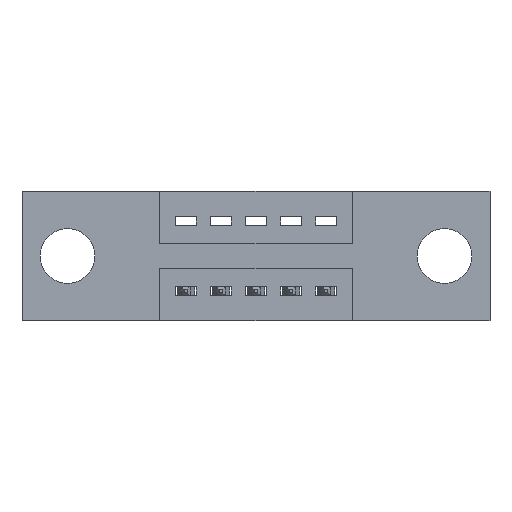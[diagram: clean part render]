
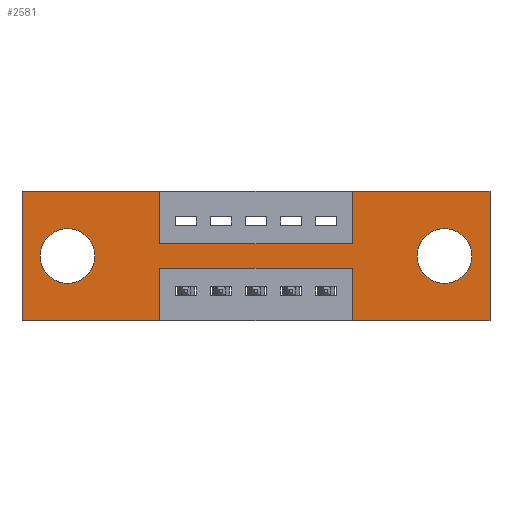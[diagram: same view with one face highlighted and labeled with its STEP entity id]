
A CAD part, front view. The second image highlights one B-rep face of the part: STEP entity #2581.
In plain terms, the highlighted planar face has unit normal (0, -1, 0).
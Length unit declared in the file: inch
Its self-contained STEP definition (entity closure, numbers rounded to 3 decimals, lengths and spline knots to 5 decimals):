
#15 = CARTESIAN_POINT ( 'NONE',  ( 0.13, 0., -0.263 ) ) ;
#109 = EDGE_CURVE ( 'NONE', #8626, #171, #8710, .T. ) ;
#113 = LINE ( 'NONE', #3577, #8083 ) ;
#143 = FACE_BOUND ( 'NONE', #386, .T. ) ;
#150 = ORIENTED_EDGE ( 'NONE', *, *, #3169, .F. ) ;
#171 = VERTEX_POINT ( 'NONE', #7213 ) ;
#253 = VERTEX_POINT ( 'NONE', #6100 ) ;
#336 = VERTEX_POINT ( 'NONE', #4728 ) ;
#356 = VERTEX_POINT ( 'NONE', #8043 ) ;
#372 = DIRECTION ( 'NONE',  ( 1., 0., 0. ) ) ;
#386 = EDGE_LOOP ( 'NONE', ( #6380, #6823 ) ) ;
#454 = VERTEX_POINT ( 'NONE', #6214 ) ;
#799 = VERTEX_POINT ( 'NONE', #6121 ) ;
#828 = LINE ( 'NONE', #1223, #1150 ) ;
#867 = ORIENTED_EDGE ( 'NONE', *, *, #2726, .F. ) ;
#883 = CARTESIAN_POINT ( 'NONE',  ( 0.9425, 0., 0. ) ) ;
#956 = DIRECTION ( 'NONE',  ( 0., 0., 1. ) ) ;
#1019 = DIRECTION ( 'NONE',  ( 0., 1., 0. ) ) ;
#1147 = CARTESIAN_POINT ( 'NONE',  ( 0.9425, 0., -0.37 ) ) ;
#1150 = VECTOR ( 'NONE', #3810, 39.37008 ) ;
#1153 = CARTESIAN_POINT ( 'NONE',  ( 0., 0., 0. ) ) ;
#1200 = AXIS2_PLACEMENT_3D ( 'NONE', #6505, #1019, #956 ) ;
#1213 = DIRECTION ( 'NONE',  ( -1., 0., 0. ) ) ;
#1223 = CARTESIAN_POINT ( 'NONE',  ( 0.3925, 0., -0.22 ) ) ;
#1631 = EDGE_CURVE ( 'NONE', #1821, #336, #8228, .T. ) ;
#1748 = CARTESIAN_POINT ( 'NONE',  ( 0., 0., 0. ) ) ;
#1821 = VERTEX_POINT ( 'NONE', #4134 ) ;
#1927 = CARTESIAN_POINT ( 'NONE',  ( 0.3925, 0., -0.22 ) ) ;
#2043 = CIRCLE ( 'NONE', #7856, 0.078 ) ;
#2061 = DIRECTION ( 'NONE',  ( 0., 0., -1. ) ) ;
#2185 = EDGE_LOOP ( 'NONE', ( #150, #3767, #7051, #867, #5070, #3225, #2313, #6167, #3788, #2284, #3753, #7090 ) ) ;
#2240 = DIRECTION ( 'NONE',  ( 0., 0., 1. ) ) ;
#2284 = ORIENTED_EDGE ( 'NONE', *, *, #5290, .F. ) ;
#2313 = ORIENTED_EDGE ( 'NONE', *, *, #2867, .F. ) ;
#2475 = VECTOR ( 'NONE', #4368, 39.37008 ) ;
#2581 = ADVANCED_FACE ( 'NONE', ( #143, #7480, #3750 ), #8185, .T. ) ;
#2722 = CARTESIAN_POINT ( 'NONE',  ( 0.3925, 0., -0.37 ) ) ;
#2726 = EDGE_CURVE ( 'NONE', #8223, #3061, #7687, .T. ) ;
#2732 = DIRECTION ( 'NONE',  ( 0., 1., 0. ) ) ;
#2829 = DIRECTION ( 'NONE',  ( 0., 0., -1. ) ) ;
#2867 = EDGE_CURVE ( 'NONE', #5758, #8626, #7140, .T. ) ;
#2986 = DIRECTION ( 'NONE',  ( 0., 0., -1. ) ) ;
#3061 = VERTEX_POINT ( 'NONE', #6664 ) ;
#3068 = LINE ( 'NONE', #3722, #8256 ) ;
#3169 = EDGE_CURVE ( 'NONE', #3504, #6821, #8399, .T. ) ;
#3225 = ORIENTED_EDGE ( 'NONE', *, *, #109, .F. ) ;
#3300 = LINE ( 'NONE', #6414, #7873 ) ;
#3504 = VERTEX_POINT ( 'NONE', #1927 ) ;
#3577 = CARTESIAN_POINT ( 'NONE',  ( 0.3925, 0., -0.15 ) ) ;
#3605 = LINE ( 'NONE', #5418, #8680 ) ;
#3722 = CARTESIAN_POINT ( 'NONE',  ( 0., 0., 0. ) ) ;
#3750 = FACE_OUTER_BOUND ( 'NONE', #2185, .T. ) ;
#3753 = ORIENTED_EDGE ( 'NONE', *, *, #7969, .F. ) ;
#3767 = ORIENTED_EDGE ( 'NONE', *, *, #8628, .F. ) ;
#3788 = ORIENTED_EDGE ( 'NONE', *, *, #4035, .F. ) ;
#3810 = DIRECTION ( 'NONE',  ( -1., 0., 0. ) ) ;
#3904 = CARTESIAN_POINT ( 'NONE',  ( 0.3925, 0., 0. ) ) ;
#3978 = VERTEX_POINT ( 'NONE', #5642 ) ;
#4035 = EDGE_CURVE ( 'NONE', #5348, #454, #3300, .T. ) ;
#4040 = EDGE_CURVE ( 'NONE', #454, #5758, #113, .T. ) ;
#4134 = CARTESIAN_POINT ( 'NONE',  ( 1.205, 0., -0.107 ) ) ;
#4186 = VECTOR ( 'NONE', #2240, 39.37008 ) ;
#4225 = AXIS2_PLACEMENT_3D ( 'NONE', #7318, #5202, #5286 ) ;
#4337 = LINE ( 'NONE', #1147, #8250 ) ;
#4368 = DIRECTION ( 'NONE',  ( 1., 0., 0. ) ) ;
#4728 = CARTESIAN_POINT ( 'NONE',  ( 1.205, 0., -0.263 ) ) ;
#4789 = EDGE_CURVE ( 'NONE', #6821, #3978, #7316, .T. ) ;
#4800 = EDGE_CURVE ( 'NONE', #171, #8223, #3605, .T. ) ;
#4844 = DIRECTION ( 'NONE',  ( 0., -1., 0. ) ) ;
#4941 = CARTESIAN_POINT ( 'NONE',  ( 0.13, 0., -0.185 ) ) ;
#5070 = ORIENTED_EDGE ( 'NONE', *, *, #4800, .F. ) ;
#5202 = DIRECTION ( 'NONE',  ( 0., 1., 0. ) ) ;
#5286 = DIRECTION ( 'NONE',  ( 0., 0., -1. ) ) ;
#5287 = CARTESIAN_POINT ( 'NONE',  ( 0., 0., -0.37 ) ) ;
#5290 = EDGE_CURVE ( 'NONE', #356, #5348, #6994, .T. ) ;
#5348 = VERTEX_POINT ( 'NONE', #3904 ) ;
#5418 = CARTESIAN_POINT ( 'NONE',  ( 1.335, 0., 0. ) ) ;
#5642 = CARTESIAN_POINT ( 'NONE',  ( 0., 0., -0.37 ) ) ;
#5758 = VERTEX_POINT ( 'NONE', #6337 ) ;
#5895 = VECTOR ( 'NONE', #1213, 39.37008 ) ;
#6072 = CIRCLE ( 'NONE', #1200, 0.078 ) ;
#6100 = CARTESIAN_POINT ( 'NONE',  ( 0.9425, 0., -0.22 ) ) ;
#6119 = CARTESIAN_POINT ( 'NONE',  ( 1.205, 0., -0.185 ) ) ;
#6121 = CARTESIAN_POINT ( 'NONE',  ( 0.13, 0., -0.107 ) ) ;
#6167 = ORIENTED_EDGE ( 'NONE', *, *, #4040, .F. ) ;
#6205 = VECTOR ( 'NONE', #2061, 39.37008 ) ;
#6214 = CARTESIAN_POINT ( 'NONE',  ( 0.3925, 0., -0.15 ) ) ;
#6236 = EDGE_LOOP ( 'NONE', ( #7913, #6737 ) ) ;
#6259 = AXIS2_PLACEMENT_3D ( 'NONE', #8208, #4844, #2829 ) ;
#6337 = CARTESIAN_POINT ( 'NONE',  ( 0.9425, 0., -0.15 ) ) ;
#6372 = DIRECTION ( 'NONE',  ( 0., 0., 1. ) ) ;
#6380 = ORIENTED_EDGE ( 'NONE', *, *, #1631, .T. ) ;
#6414 = CARTESIAN_POINT ( 'NONE',  ( 0.3925, 0., 0. ) ) ;
#6439 = DIRECTION ( 'NONE',  ( 0., 0., 1. ) ) ;
#6479 = VERTEX_POINT ( 'NONE', #15 ) ;
#6505 = CARTESIAN_POINT ( 'NONE',  ( 0.13, 0., -0.185 ) ) ;
#6621 = EDGE_CURVE ( 'NONE', #6479, #799, #2043, .T. ) ;
#6664 = CARTESIAN_POINT ( 'NONE',  ( 0.9425, 0., -0.37 ) ) ;
#6737 = ORIENTED_EDGE ( 'NONE', *, *, #6621, .T. ) ;
#6821 = VERTEX_POINT ( 'NONE', #7899 ) ;
#6823 = ORIENTED_EDGE ( 'NONE', *, *, #8340, .T. ) ;
#6994 = LINE ( 'NONE', #1153, #8464 ) ;
#7051 = ORIENTED_EDGE ( 'NONE', *, *, #8147, .F. ) ;
#7059 = EDGE_CURVE ( 'NONE', #799, #6479, #6072, .T. ) ;
#7090 = ORIENTED_EDGE ( 'NONE', *, *, #4789, .F. ) ;
#7140 = LINE ( 'NONE', #883, #4186 ) ;
#7213 = CARTESIAN_POINT ( 'NONE',  ( 1.335, 0., 0. ) ) ;
#7316 = LINE ( 'NONE', #8646, #8169 ) ;
#7318 = CARTESIAN_POINT ( 'NONE',  ( 1.205, 0., -0.185 ) ) ;
#7384 = DIRECTION ( 'NONE',  ( -1., 0., 0. ) ) ;
#7415 = DIRECTION ( 'NONE',  ( 0., 0., -1. ) ) ;
#7474 = DIRECTION ( 'NONE',  ( 0., 0., -1. ) ) ;
#7480 = FACE_BOUND ( 'NONE', #6236, .T. ) ;
#7590 = AXIS2_PLACEMENT_3D ( 'NONE', #6119, #2732, #7474 ) ;
#7632 = DIRECTION ( 'NONE',  ( 0., 1., 0. ) ) ;
#7687 = LINE ( 'NONE', #5287, #5895 ) ;
#7856 = AXIS2_PLACEMENT_3D ( 'NONE', #4941, #7632, #6372 ) ;
#7873 = VECTOR ( 'NONE', #2986, 39.37008 ) ;
#7899 = CARTESIAN_POINT ( 'NONE',  ( 0.3925, 0., -0.37 ) ) ;
#7913 = ORIENTED_EDGE ( 'NONE', *, *, #7059, .T. ) ;
#7969 = EDGE_CURVE ( 'NONE', #3978, #356, #3068, .T. ) ;
#7984 = CARTESIAN_POINT ( 'NONE',  ( 0.9425, 0., 0. ) ) ;
#8043 = CARTESIAN_POINT ( 'NONE',  ( 0., 0., 0. ) ) ;
#8053 = CARTESIAN_POINT ( 'NONE',  ( 1.335, 0., -0.37 ) ) ;
#8083 = VECTOR ( 'NONE', #8307, 39.37008 ) ;
#8147 = EDGE_CURVE ( 'NONE', #3061, #253, #4337, .T. ) ;
#8169 = VECTOR ( 'NONE', #7384, 39.37008 ) ;
#8185 = PLANE ( 'NONE',  #6259 ) ;
#8208 = CARTESIAN_POINT ( 'NONE',  ( 0., 0., -0.37 ) ) ;
#8223 = VERTEX_POINT ( 'NONE', #8053 ) ;
#8228 = CIRCLE ( 'NONE', #7590, 0.078 ) ;
#8250 = VECTOR ( 'NONE', #8509, 39.37008 ) ;
#8256 = VECTOR ( 'NONE', #6439, 39.37008 ) ;
#8307 = DIRECTION ( 'NONE',  ( 1., 0., 0. ) ) ;
#8340 = EDGE_CURVE ( 'NONE', #336, #1821, #8342, .T. ) ;
#8342 = CIRCLE ( 'NONE', #4225, 0.078 ) ;
#8399 = LINE ( 'NONE', #2722, #6205 ) ;
#8464 = VECTOR ( 'NONE', #372, 39.37008 ) ;
#8509 = DIRECTION ( 'NONE',  ( 0., 0., 1. ) ) ;
#8626 = VERTEX_POINT ( 'NONE', #7984 ) ;
#8628 = EDGE_CURVE ( 'NONE', #253, #3504, #828, .T. ) ;
#8646 = CARTESIAN_POINT ( 'NONE',  ( 0., 0., -0.37 ) ) ;
#8680 = VECTOR ( 'NONE', #7415, 39.37008 ) ;
#8710 = LINE ( 'NONE', #1748, #2475 ) ;
